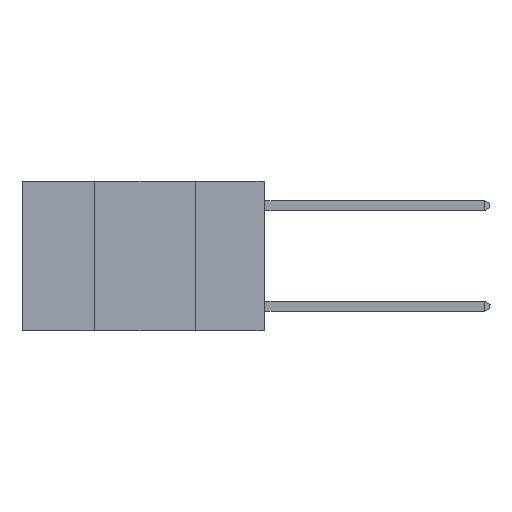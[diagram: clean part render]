
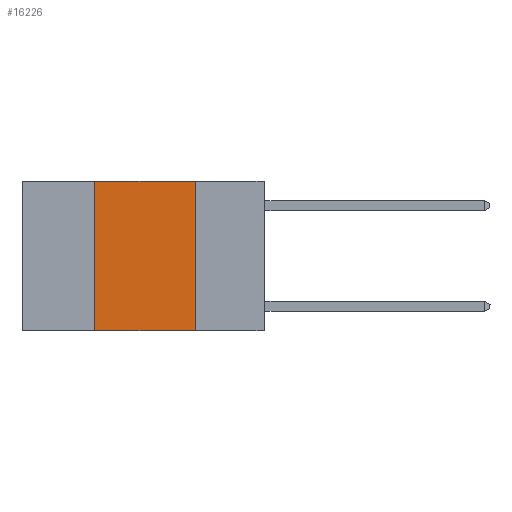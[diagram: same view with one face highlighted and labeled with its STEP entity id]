
A CAD part, left-side view. The second image highlights one B-rep face of the part: STEP entity #16226.
In plain terms, the highlighted planar face has unit normal (-1, 0, 0).
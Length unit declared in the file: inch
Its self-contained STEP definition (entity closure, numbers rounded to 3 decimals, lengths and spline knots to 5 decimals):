
#720 = VERTEX_POINT ( 'NONE', #9500 ) ;
#1154 = LINE ( 'NONE', #11971, #3173 ) ;
#1224 = DIRECTION ( 'NONE',  ( 0., 0., -1. ) ) ;
#1350 = VECTOR ( 'NONE', #15769, 39.37008 ) ;
#1451 = CARTESIAN_POINT ( 'NONE',  ( 0., 0.42, 0. ) ) ;
#2289 = EDGE_CURVE ( 'NONE', #6032, #15351, #11367, .T. ) ;
#2901 = DIRECTION ( 'NONE',  ( 1., 0., 0. ) ) ;
#3173 = VECTOR ( 'NONE', #14674, 39.37008 ) ;
#4793 = ORIENTED_EDGE ( 'NONE', *, *, #14219, .F. ) ;
#5001 = CARTESIAN_POINT ( 'NONE',  ( 0., 0.17, 0. ) ) ;
#5384 = VERTEX_POINT ( 'NONE', #1451 ) ;
#5495 = CARTESIAN_POINT ( 'NONE',  ( 0., 0.6, 0. ) ) ;
#6032 = VERTEX_POINT ( 'NONE', #13410 ) ;
#6059 = EDGE_LOOP ( 'NONE', ( #14103, #4793, #9547, #16689 ) ) ;
#6121 = CARTESIAN_POINT ( 'NONE',  ( 0., 0.6, -0.37 ) ) ;
#6562 = CARTESIAN_POINT ( 'NONE',  ( 0., 0.6, 0. ) ) ;
#7870 = AXIS2_PLACEMENT_3D ( 'NONE', #5495, #2901, #11191 ) ;
#9354 = EDGE_CURVE ( 'NONE', #6032, #5384, #1154, .T. ) ;
#9500 = CARTESIAN_POINT ( 'NONE',  ( 0., 0.17, 0. ) ) ;
#9529 = VECTOR ( 'NONE', #11991, 39.37008 ) ;
#9547 = ORIENTED_EDGE ( 'NONE', *, *, #9354, .F. ) ;
#9928 = EDGE_CURVE ( 'NONE', #720, #15351, #17368, .T. ) ;
#11013 = FACE_OUTER_BOUND ( 'NONE', #6059, .T. ) ;
#11191 = DIRECTION ( 'NONE',  ( 0., 0., -1. ) ) ;
#11367 = LINE ( 'NONE', #6121, #1350 ) ;
#11971 = CARTESIAN_POINT ( 'NONE',  ( 0., 0.42, 0. ) ) ;
#11991 = DIRECTION ( 'NONE',  ( 0., -1., 0. ) ) ;
#13270 = CARTESIAN_POINT ( 'NONE',  ( 0., 0.17, -0.37 ) ) ;
#13410 = CARTESIAN_POINT ( 'NONE',  ( 0., 0.42, -0.37 ) ) ;
#13739 = PLANE ( 'NONE',  #7870 ) ;
#13807 = LINE ( 'NONE', #6562, #9529 ) ;
#14103 = ORIENTED_EDGE ( 'NONE', *, *, #9928, .F. ) ;
#14219 = EDGE_CURVE ( 'NONE', #5384, #720, #13807, .T. ) ;
#14674 = DIRECTION ( 'NONE',  ( 0., 0., 1. ) ) ;
#15351 = VERTEX_POINT ( 'NONE', #13270 ) ;
#15769 = DIRECTION ( 'NONE',  ( 0., -1., 0. ) ) ;
#16030 = VECTOR ( 'NONE', #1224, 39.37008 ) ;
#16226 = ADVANCED_FACE ( 'NONE', ( #11013 ), #13739, .F. ) ;
#16689 = ORIENTED_EDGE ( 'NONE', *, *, #2289, .T. ) ;
#17368 = LINE ( 'NONE', #5001, #16030 ) ;
